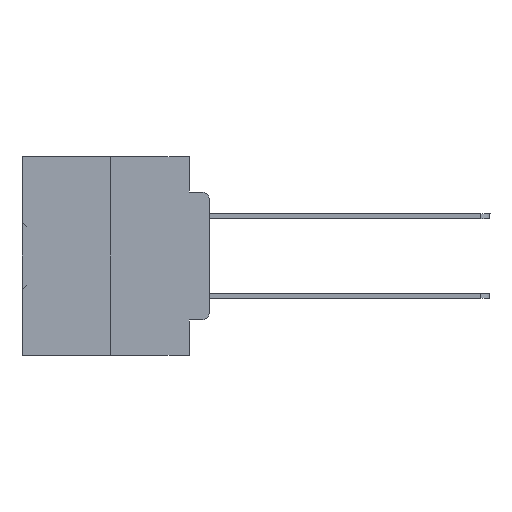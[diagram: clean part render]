
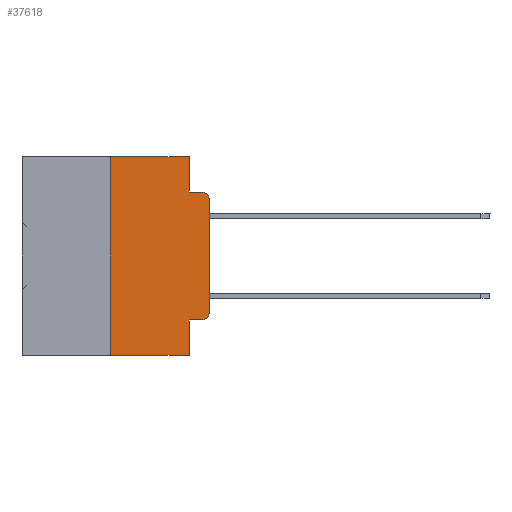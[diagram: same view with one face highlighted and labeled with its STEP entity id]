
A CAD part, left-side view. The second image highlights one B-rep face of the part: STEP entity #37618.
In plain terms, the highlighted planar face has unit normal (-1, 0, 0).
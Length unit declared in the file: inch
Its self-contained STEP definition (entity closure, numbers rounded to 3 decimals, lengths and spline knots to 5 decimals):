
#486 = VERTEX_POINT ( 'NONE', #1480 ) ;
#943 = EDGE_LOOP ( 'NONE', ( #21937, #1122, #12544, #33050, #18669, #16571, #1252, #36515, #28886, #20360 ) ) ;
#952 = AXIS2_PLACEMENT_3D ( 'NONE', #6884, #10624, #33478 ) ;
#1122 = ORIENTED_EDGE ( 'NONE', *, *, #16043, .T. ) ;
#1159 = CARTESIAN_POINT ( 'NONE',  ( 0., 0., -0.3915 ) ) ;
#1252 = ORIENTED_EDGE ( 'NONE', *, *, #35530, .T. ) ;
#1378 = CARTESIAN_POINT ( 'NONE',  ( 0., 0.25, -0.5 ) ) ;
#1480 = CARTESIAN_POINT ( 'NONE',  ( 0., 0.25, 0. ) ) ;
#1495 = CARTESIAN_POINT ( 'NONE',  ( 0., 0.02, -0.0885 ) ) ;
#3235 = CARTESIAN_POINT ( 'NONE',  ( 0., 0.02, -0.4115 ) ) ;
#3936 = CARTESIAN_POINT ( 'NONE',  ( 0., 0.25, 0. ) ) ;
#4521 = DIRECTION ( 'NONE',  ( 1., 0., 0. ) ) ;
#5212 = CARTESIAN_POINT ( 'NONE',  ( 0., 0.473, 0. ) ) ;
#5419 = DIRECTION ( 'NONE',  ( 0., -1., 0. ) ) ;
#5483 = EDGE_CURVE ( 'NONE', #486, #20793, #8717, .T. ) ;
#5505 = LINE ( 'NONE', #34500, #8715 ) ;
#6884 = CARTESIAN_POINT ( 'NONE',  ( 0., 0.02, -0.1085 ) ) ;
#6920 = DIRECTION ( 'NONE',  ( 0., -1., 0. ) ) ;
#7083 = AXIS2_PLACEMENT_3D ( 'NONE', #22529, #25215, #16128 ) ;
#7121 = PLANE ( 'NONE',  #16736 ) ;
#7990 = CARTESIAN_POINT ( 'NONE',  ( 0., 0.051, 0. ) ) ;
#8254 = CARTESIAN_POINT ( 'NONE',  ( 0., 0.051, -0.0885 ) ) ;
#8543 = VERTEX_POINT ( 'NONE', #1159 ) ;
#8715 = VECTOR ( 'NONE', #20300, 39.37008 ) ;
#8717 = LINE ( 'NONE', #5212, #18494 ) ;
#8824 = VERTEX_POINT ( 'NONE', #28907 ) ;
#8938 = CIRCLE ( 'NONE', #952, 0.02 ) ;
#10624 = DIRECTION ( 'NONE',  ( -1., 0., 0. ) ) ;
#10735 = VERTEX_POINT ( 'NONE', #26054 ) ;
#11169 = DIRECTION ( 'NONE',  ( 0., -1., 0. ) ) ;
#11301 = DIRECTION ( 'NONE',  ( 0., 0., 1. ) ) ;
#12475 = EDGE_CURVE ( 'NONE', #8543, #8824, #19456, .T. ) ;
#12544 = ORIENTED_EDGE ( 'NONE', *, *, #16903, .F. ) ;
#15483 = CARTESIAN_POINT ( 'NONE',  ( 0., 0.051, -0.4115 ) ) ;
#15656 = CARTESIAN_POINT ( 'NONE',  ( 0., 0.051, -0.4115 ) ) ;
#15737 = VECTOR ( 'NONE', #11301, 39.37008 ) ;
#15954 = VERTEX_POINT ( 'NONE', #3235 ) ;
#16043 = EDGE_CURVE ( 'NONE', #8824, #30989, #8938, .T. ) ;
#16128 = DIRECTION ( 'NONE',  ( 0., 0., -1. ) ) ;
#16571 = ORIENTED_EDGE ( 'NONE', *, *, #28277, .F. ) ;
#16736 = AXIS2_PLACEMENT_3D ( 'NONE', #19575, #4521, #34243 ) ;
#16903 = EDGE_CURVE ( 'NONE', #10735, #30989, #24204, .T. ) ;
#17464 = LINE ( 'NONE', #25825, #25361 ) ;
#18112 = CIRCLE ( 'NONE', #7083, 0.02 ) ;
#18400 = FACE_OUTER_BOUND ( 'NONE', #943, .T. ) ;
#18494 = VECTOR ( 'NONE', #11169, 39.37008 ) ;
#18669 = ORIENTED_EDGE ( 'NONE', *, *, #5483, .F. ) ;
#19456 = LINE ( 'NONE', #25999, #15737 ) ;
#19575 = CARTESIAN_POINT ( 'NONE',  ( 0., 0.473, 0. ) ) ;
#20300 = DIRECTION ( 'NONE',  ( 0., -1., 0. ) ) ;
#20360 = ORIENTED_EDGE ( 'NONE', *, *, #23489, .T. ) ;
#20638 = VERTEX_POINT ( 'NONE', #1378 ) ;
#20793 = VERTEX_POINT ( 'NONE', #34830 ) ;
#21937 = ORIENTED_EDGE ( 'NONE', *, *, #12475, .T. ) ;
#22157 = LINE ( 'NONE', #7990, #36983 ) ;
#22401 = VERTEX_POINT ( 'NONE', #15656 ) ;
#22529 = CARTESIAN_POINT ( 'NONE',  ( 0., 0.02, -0.3915 ) ) ;
#22974 = DIRECTION ( 'NONE',  ( 0., 0., -1. ) ) ;
#23489 = EDGE_CURVE ( 'NONE', #15954, #8543, #18112, .T. ) ;
#24204 = LINE ( 'NONE', #8254, #32045 ) ;
#25215 = DIRECTION ( 'NONE',  ( -1., 0., 0. ) ) ;
#25361 = VECTOR ( 'NONE', #22974, 39.37008 ) ;
#25825 = CARTESIAN_POINT ( 'NONE',  ( 0., 0.051, 0. ) ) ;
#25999 = CARTESIAN_POINT ( 'NONE',  ( 0., 0., 0. ) ) ;
#26054 = CARTESIAN_POINT ( 'NONE',  ( 0., 0.051, -0.0885 ) ) ;
#26388 = EDGE_CURVE ( 'NONE', #22401, #15954, #37399, .T. ) ;
#28277 = EDGE_CURVE ( 'NONE', #20638, #486, #32579, .T. ) ;
#28767 = DIRECTION ( 'NONE',  ( 0., 0., -1. ) ) ;
#28886 = ORIENTED_EDGE ( 'NONE', *, *, #26388, .T. ) ;
#28907 = CARTESIAN_POINT ( 'NONE',  ( 0., 0., -0.1085 ) ) ;
#30407 = VECTOR ( 'NONE', #6920, 39.37008 ) ;
#30562 = DIRECTION ( 'NONE',  ( 0., 0., 1. ) ) ;
#30989 = VERTEX_POINT ( 'NONE', #1495 ) ;
#31768 = CARTESIAN_POINT ( 'NONE',  ( 0., 0.051, -0.5 ) ) ;
#32045 = VECTOR ( 'NONE', #5419, 39.37008 ) ;
#32579 = LINE ( 'NONE', #3936, #35392 ) ;
#33050 = ORIENTED_EDGE ( 'NONE', *, *, #36855, .F. ) ;
#33478 = DIRECTION ( 'NONE',  ( 0., 0., -1. ) ) ;
#34243 = DIRECTION ( 'NONE',  ( 0., 0., -1. ) ) ;
#34500 = CARTESIAN_POINT ( 'NONE',  ( 0., 0.473, -0.5 ) ) ;
#34830 = CARTESIAN_POINT ( 'NONE',  ( 0., 0.051, 0. ) ) ;
#35392 = VECTOR ( 'NONE', #30562, 39.37008 ) ;
#35530 = EDGE_CURVE ( 'NONE', #20638, #37734, #5505, .T. ) ;
#36515 = ORIENTED_EDGE ( 'NONE', *, *, #37775, .F. ) ;
#36855 = EDGE_CURVE ( 'NONE', #20793, #10735, #22157, .T. ) ;
#36983 = VECTOR ( 'NONE', #28767, 39.37008 ) ;
#37399 = LINE ( 'NONE', #15483, #30407 ) ;
#37618 = ADVANCED_FACE ( 'NONE', ( #18400 ), #7121, .F. ) ;
#37734 = VERTEX_POINT ( 'NONE', #31768 ) ;
#37775 = EDGE_CURVE ( 'NONE', #22401, #37734, #17464, .T. ) ;
